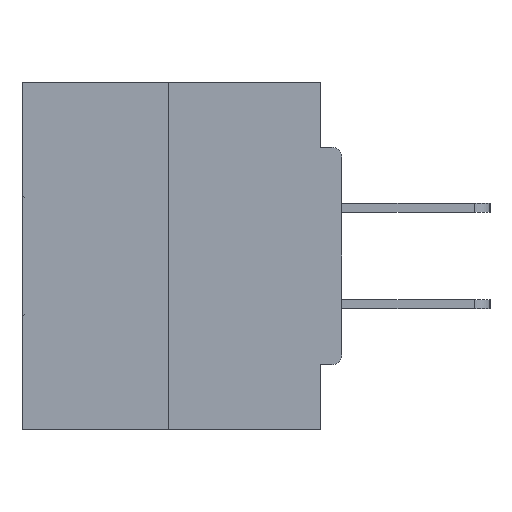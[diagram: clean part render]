
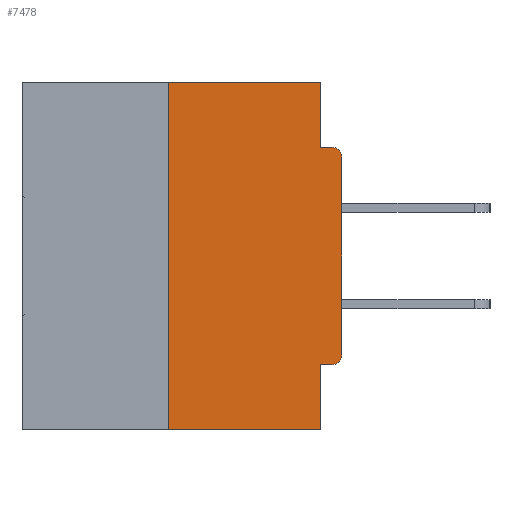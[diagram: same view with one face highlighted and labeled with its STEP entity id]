
A CAD part, left-side view. The second image highlights one B-rep face of the part: STEP entity #7478.
In plain terms, the highlighted planar face has unit normal (-1, 0, 0).
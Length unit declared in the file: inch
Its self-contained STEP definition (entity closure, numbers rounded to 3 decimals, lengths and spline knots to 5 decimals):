
#326 = VERTEX_POINT ( 'NONE', #13112 ) ;
#360 = CIRCLE ( 'NONE', #30986, 0.015 ) ;
#560 = VERTEX_POINT ( 'NONE', #1074 ) ;
#740 = DIRECTION ( 'NONE',  ( 1., 0., 0. ) ) ;
#1074 = CARTESIAN_POINT ( 'NONE',  ( 0., 0.031, -0.5 ) ) ;
#1280 = VERTEX_POINT ( 'NONE', #17449 ) ;
#1636 = CARTESIAN_POINT ( 'NONE',  ( 0., 0.031, -0.5 ) ) ;
#1685 = LINE ( 'NONE', #19870, #12203 ) ;
#1792 = VECTOR ( 'NONE', #28431, 39.37008 ) ;
#2228 = ORIENTED_EDGE ( 'NONE', *, *, #19136, .F. ) ;
#2941 = ORIENTED_EDGE ( 'NONE', *, *, #20505, .F. ) ;
#4290 = DIRECTION ( 'NONE',  ( 0., 0., -1. ) ) ;
#4292 = DIRECTION ( 'NONE',  ( 0., 0., -1. ) ) ;
#4441 = LINE ( 'NONE', #8898, #40937 ) ;
#4630 = CARTESIAN_POINT ( 'NONE',  ( 0., 0., -0.3915 ) ) ;
#4727 = VERTEX_POINT ( 'NONE', #26427 ) ;
#4764 = VECTOR ( 'NONE', #4794, 39.37008 ) ;
#4794 = DIRECTION ( 'NONE',  ( 0., 0., 1. ) ) ;
#4829 = EDGE_LOOP ( 'NONE', ( #9634, #2228, #29741, #2941, #20632, #38616, #23377, #7417, #7828, #30999 ) ) ;
#6051 = CARTESIAN_POINT ( 'NONE',  ( 0., 0., 0. ) ) ;
#7417 = ORIENTED_EDGE ( 'NONE', *, *, #13595, .T. ) ;
#7478 = ADVANCED_FACE ( 'NONE', ( #39619 ), #26493, .F. ) ;
#7828 = ORIENTED_EDGE ( 'NONE', *, *, #18400, .F. ) ;
#7842 = LINE ( 'NONE', #6051, #1792 ) ;
#8898 = CARTESIAN_POINT ( 'NONE',  ( 0., 0.031, 0. ) ) ;
#9634 = ORIENTED_EDGE ( 'NONE', *, *, #26232, .F. ) ;
#11432 = LINE ( 'NONE', #40086, #32964 ) ;
#11823 = CARTESIAN_POINT ( 'NONE',  ( 0., 0.015, -0.0935 ) ) ;
#12203 = VECTOR ( 'NONE', #13124, 39.37008 ) ;
#13112 = CARTESIAN_POINT ( 'NONE',  ( 0., 0.25, 0. ) ) ;
#13124 = DIRECTION ( 'NONE',  ( 0., -1., 0. ) ) ;
#13316 = VERTEX_POINT ( 'NONE', #21835 ) ;
#13595 = EDGE_CURVE ( 'NONE', #4727, #38503, #31946, .T. ) ;
#13983 = EDGE_CURVE ( 'NONE', #33916, #18716, #360, .T. ) ;
#14757 = AXIS2_PLACEMENT_3D ( 'NONE', #26360, #740, #4292 ) ;
#14811 = VERTEX_POINT ( 'NONE', #31818 ) ;
#15467 = CARTESIAN_POINT ( 'NONE',  ( 0., 0.015, -0.3915 ) ) ;
#16082 = VECTOR ( 'NONE', #40549, 39.37008 ) ;
#17260 = EDGE_CURVE ( 'NONE', #33916, #40350, #30382, .T. ) ;
#17449 = CARTESIAN_POINT ( 'NONE',  ( 0., 0.25, -0.5 ) ) ;
#18095 = DIRECTION ( 'NONE',  ( 0., -1., 0. ) ) ;
#18400 = EDGE_CURVE ( 'NONE', #13316, #38503, #40868, .T. ) ;
#18412 = EDGE_CURVE ( 'NONE', #18716, #4727, #7842, .T. ) ;
#18716 = VERTEX_POINT ( 'NONE', #4630 ) ;
#19136 = EDGE_CURVE ( 'NONE', #1280, #326, #21764, .T. ) ;
#19870 = CARTESIAN_POINT ( 'NONE',  ( 0., 0.46, 0. ) ) ;
#20505 = EDGE_CURVE ( 'NONE', #40350, #560, #39142, .T. ) ;
#20632 = ORIENTED_EDGE ( 'NONE', *, *, #17260, .F. ) ;
#21764 = LINE ( 'NONE', #27288, #4764 ) ;
#21835 = CARTESIAN_POINT ( 'NONE',  ( 0., 0.031, -0.0935 ) ) ;
#22025 = DIRECTION ( 'NONE',  ( 0., -1., 0. ) ) ;
#22777 = EDGE_CURVE ( 'NONE', #14811, #13316, #4441, .T. ) ;
#23036 = DIRECTION ( 'NONE',  ( 0., 0., -1. ) ) ;
#23377 = ORIENTED_EDGE ( 'NONE', *, *, #18412, .T. ) ;
#25570 = DIRECTION ( 'NONE',  ( 0., 1., 0. ) ) ;
#26232 = EDGE_CURVE ( 'NONE', #326, #14811, #1685, .T. ) ;
#26360 = CARTESIAN_POINT ( 'NONE',  ( 0., 0.46, 0. ) ) ;
#26427 = CARTESIAN_POINT ( 'NONE',  ( 0., 0., -0.1085 ) ) ;
#26493 = PLANE ( 'NONE',  #14757 ) ;
#27288 = CARTESIAN_POINT ( 'NONE',  ( 0., 0.25, 0. ) ) ;
#28190 = DIRECTION ( 'NONE',  ( -1., 0., 0. ) ) ;
#28431 = DIRECTION ( 'NONE',  ( 0., 0., 1. ) ) ;
#28467 = DIRECTION ( 'NONE',  ( 0., 0., -1. ) ) ;
#29442 = CARTESIAN_POINT ( 'NONE',  ( 0., 0.015, -0.1085 ) ) ;
#29741 = ORIENTED_EDGE ( 'NONE', *, *, #39050, .T. ) ;
#29869 = DIRECTION ( 'NONE',  ( -1., 0., 0. ) ) ;
#30382 = LINE ( 'NONE', #38157, #35852 ) ;
#30554 = CARTESIAN_POINT ( 'NONE',  ( 0., 0.031, -0.4065 ) ) ;
#30986 = AXIS2_PLACEMENT_3D ( 'NONE', #15467, #28190, #28467 ) ;
#30999 = ORIENTED_EDGE ( 'NONE', *, *, #22777, .F. ) ;
#31411 = CARTESIAN_POINT ( 'NONE',  ( 0., 0.015, -0.4065 ) ) ;
#31818 = CARTESIAN_POINT ( 'NONE',  ( 0., 0.031, 0. ) ) ;
#31946 = CIRCLE ( 'NONE', #40156, 0.015 ) ;
#32964 = VECTOR ( 'NONE', #18095, 39.37008 ) ;
#33916 = VERTEX_POINT ( 'NONE', #31411 ) ;
#35852 = VECTOR ( 'NONE', #25570, 39.37008 ) ;
#38157 = CARTESIAN_POINT ( 'NONE',  ( 0., 0., -0.4065 ) ) ;
#38211 = CARTESIAN_POINT ( 'NONE',  ( 0., 0., -0.0935 ) ) ;
#38503 = VERTEX_POINT ( 'NONE', #11823 ) ;
#38616 = ORIENTED_EDGE ( 'NONE', *, *, #13983, .T. ) ;
#39050 = EDGE_CURVE ( 'NONE', #1280, #560, #11432, .T. ) ;
#39142 = LINE ( 'NONE', #1636, #16082 ) ;
#39619 = FACE_OUTER_BOUND ( 'NONE', #4829, .T. ) ;
#40086 = CARTESIAN_POINT ( 'NONE',  ( 0., 0.46, -0.5 ) ) ;
#40156 = AXIS2_PLACEMENT_3D ( 'NONE', #29442, #29869, #4290 ) ;
#40350 = VERTEX_POINT ( 'NONE', #30554 ) ;
#40363 = VECTOR ( 'NONE', #22025, 39.37008 ) ;
#40549 = DIRECTION ( 'NONE',  ( 0., 0., -1. ) ) ;
#40868 = LINE ( 'NONE', #38211, #40363 ) ;
#40937 = VECTOR ( 'NONE', #23036, 39.37008 ) ;
